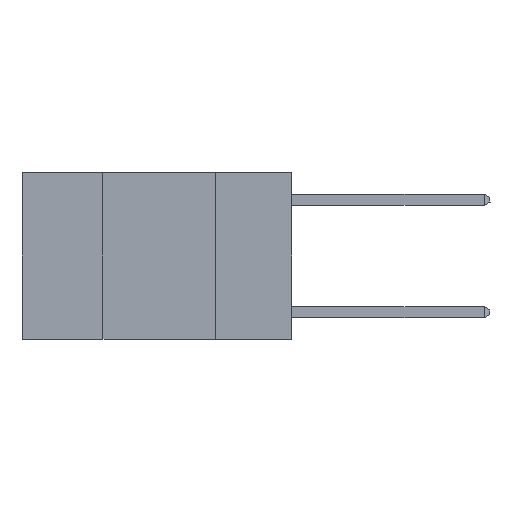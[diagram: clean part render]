
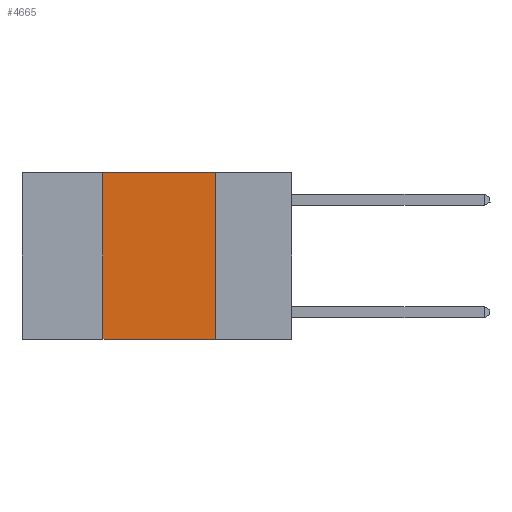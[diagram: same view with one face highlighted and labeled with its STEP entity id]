
A CAD part, left-side view. The second image highlights one B-rep face of the part: STEP entity #4665.
In plain terms, the highlighted planar face has unit normal (-1, 0, 0).
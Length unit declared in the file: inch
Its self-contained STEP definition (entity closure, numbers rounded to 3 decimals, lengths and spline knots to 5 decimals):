
#775 = DIRECTION ( 'NONE',  ( 0., 0., -1. ) ) ;
#837 = LINE ( 'NONE', #9460, #8116 ) ;
#936 = DIRECTION ( 'NONE',  ( 0., -1., 0. ) ) ;
#1879 = CARTESIAN_POINT ( 'NONE',  ( 0., 0.6, 0. ) ) ;
#2092 = VERTEX_POINT ( 'NONE', #8807 ) ;
#2181 = CARTESIAN_POINT ( 'NONE',  ( 0., 0.6, -0.37 ) ) ;
#2340 = DIRECTION ( 'NONE',  ( 0., 0., -1. ) ) ;
#3798 = EDGE_CURVE ( 'NONE', #9395, #2092, #9063, .T. ) ;
#4058 = DIRECTION ( 'NONE',  ( 0., 0., 1. ) ) ;
#4348 = LINE ( 'NONE', #6906, #8840 ) ;
#4378 = ORIENTED_EDGE ( 'NONE', *, *, #9472, .F. ) ;
#4399 = VERTEX_POINT ( 'NONE', #5054 ) ;
#4440 = PLANE ( 'NONE',  #10499 ) ;
#4663 = ORIENTED_EDGE ( 'NONE', *, *, #11187, .F. ) ;
#4665 = ADVANCED_FACE ( 'NONE', ( #9043 ), #4440, .F. ) ;
#5054 = CARTESIAN_POINT ( 'NONE',  ( 0., 0.17, 0. ) ) ;
#6268 = DIRECTION ( 'NONE',  ( 1., 0., 0. ) ) ;
#6691 = VECTOR ( 'NONE', #9427, 39.37008 ) ;
#6906 = CARTESIAN_POINT ( 'NONE',  ( 0., 0.17, 0. ) ) ;
#7073 = ORIENTED_EDGE ( 'NONE', *, *, #3798, .T. ) ;
#7336 = CARTESIAN_POINT ( 'NONE',  ( 0., 0.42, 0. ) ) ;
#8030 = CARTESIAN_POINT ( 'NONE',  ( 0., 0.6, 0. ) ) ;
#8116 = VECTOR ( 'NONE', #4058, 39.37008 ) ;
#8673 = VECTOR ( 'NONE', #936, 39.37008 ) ;
#8807 = CARTESIAN_POINT ( 'NONE',  ( 0., 0.17, -0.37 ) ) ;
#8840 = VECTOR ( 'NONE', #2340, 39.37008 ) ;
#9043 = FACE_OUTER_BOUND ( 'NONE', #10031, .T. ) ;
#9063 = LINE ( 'NONE', #2181, #6691 ) ;
#9098 = VERTEX_POINT ( 'NONE', #7336 ) ;
#9119 = EDGE_CURVE ( 'NONE', #9098, #4399, #10986, .T. ) ;
#9157 = ORIENTED_EDGE ( 'NONE', *, *, #9119, .F. ) ;
#9395 = VERTEX_POINT ( 'NONE', #10361 ) ;
#9427 = DIRECTION ( 'NONE',  ( 0., -1., 0. ) ) ;
#9460 = CARTESIAN_POINT ( 'NONE',  ( 0., 0.42, 0. ) ) ;
#9472 = EDGE_CURVE ( 'NONE', #4399, #2092, #4348, .T. ) ;
#10031 = EDGE_LOOP ( 'NONE', ( #4378, #9157, #4663, #7073 ) ) ;
#10361 = CARTESIAN_POINT ( 'NONE',  ( 0., 0.42, -0.37 ) ) ;
#10499 = AXIS2_PLACEMENT_3D ( 'NONE', #8030, #6268, #775 ) ;
#10986 = LINE ( 'NONE', #1879, #8673 ) ;
#11187 = EDGE_CURVE ( 'NONE', #9395, #9098, #837, .T. ) ;
